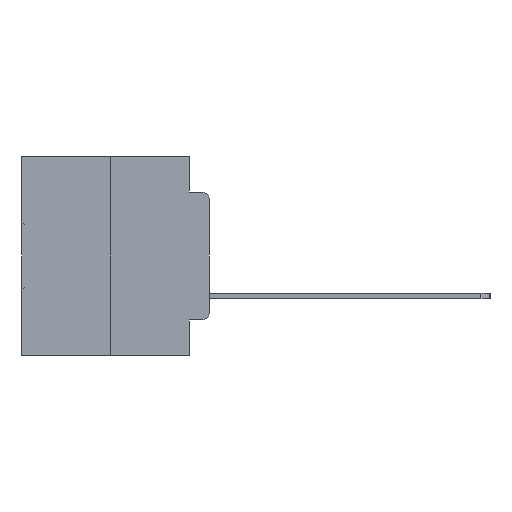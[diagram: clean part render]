
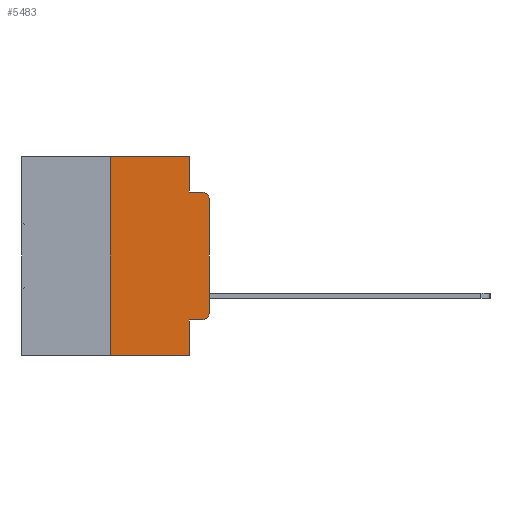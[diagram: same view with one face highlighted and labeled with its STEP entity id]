
A CAD part, left-side view. The second image highlights one B-rep face of the part: STEP entity #5483.
In plain terms, the highlighted planar face has unit normal (-1, 0, 0).
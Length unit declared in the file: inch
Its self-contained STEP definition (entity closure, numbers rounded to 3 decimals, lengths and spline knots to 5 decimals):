
#379 = DIRECTION ( 'NONE',  ( 0., 0., 1. ) ) ;
#592 = ORIENTED_EDGE ( 'NONE', *, *, #28308, .F. ) ;
#1482 = VERTEX_POINT ( 'NONE', #16239 ) ;
#1504 = VECTOR ( 'NONE', #26684, 39.37008 ) ;
#1857 = CARTESIAN_POINT ( 'NONE',  ( 0., 0.25, 0. ) ) ;
#3436 = VECTOR ( 'NONE', #13293, 39.37008 ) ;
#3845 = VECTOR ( 'NONE', #379, 39.37008 ) ;
#4010 = CARTESIAN_POINT ( 'NONE',  ( 0., 0.051, -0.4115 ) ) ;
#4102 = ORIENTED_EDGE ( 'NONE', *, *, #18301, .T. ) ;
#4181 = CARTESIAN_POINT ( 'NONE',  ( 0., 0.473, -0.5 ) ) ;
#4289 = AXIS2_PLACEMENT_3D ( 'NONE', #13052, #29774, #15468 ) ;
#4316 = VERTEX_POINT ( 'NONE', #24031 ) ;
#4359 = EDGE_CURVE ( 'NONE', #24168, #29425, #23856, .T. ) ;
#4875 = PLANE ( 'NONE',  #23037 ) ;
#5258 = VECTOR ( 'NONE', #10663, 39.37008 ) ;
#5371 = LINE ( 'NONE', #11793, #17595 ) ;
#5483 = ADVANCED_FACE ( 'NONE', ( #25859 ), #4875, .F. ) ;
#6057 = EDGE_CURVE ( 'NONE', #1482, #29607, #23603, .T. ) ;
#6245 = EDGE_CURVE ( 'NONE', #4316, #14714, #10385, .T. ) ;
#7297 = CARTESIAN_POINT ( 'NONE',  ( 0., 0.051, -0.5 ) ) ;
#7557 = ORIENTED_EDGE ( 'NONE', *, *, #7848, .T. ) ;
#7736 = CARTESIAN_POINT ( 'NONE',  ( 0., 0.25, 0. ) ) ;
#7848 = EDGE_CURVE ( 'NONE', #23346, #29607, #15579, .T. ) ;
#9597 = CARTESIAN_POINT ( 'NONE',  ( 0., 0.051, -0.0885 ) ) ;
#9608 = CARTESIAN_POINT ( 'NONE',  ( 0., 0.02, -0.1085 ) ) ;
#9739 = EDGE_LOOP ( 'NONE', ( #4102, #7557, #12170, #11010, #592, #30859, #26072, #15923, #17452, #18971 ) ) ;
#9835 = DIRECTION ( 'NONE',  ( 1., 0., 0. ) ) ;
#10385 = LINE ( 'NONE', #7736, #3845 ) ;
#10663 = DIRECTION ( 'NONE',  ( 0., -1., 0. ) ) ;
#10708 = CARTESIAN_POINT ( 'NONE',  ( 0., 0., -0.1085 ) ) ;
#10849 = CARTESIAN_POINT ( 'NONE',  ( 0., 0., 0. ) ) ;
#11010 = ORIENTED_EDGE ( 'NONE', *, *, #14440, .F. ) ;
#11793 = CARTESIAN_POINT ( 'NONE',  ( 0., 0.473, 0. ) ) ;
#11798 = AXIS2_PLACEMENT_3D ( 'NONE', #9608, #26420, #12046 ) ;
#12046 = DIRECTION ( 'NONE',  ( 0., 0., -1. ) ) ;
#12170 = ORIENTED_EDGE ( 'NONE', *, *, #6057, .F. ) ;
#12896 = EDGE_CURVE ( 'NONE', #4316, #21151, #26655, .T. ) ;
#13052 = CARTESIAN_POINT ( 'NONE',  ( 0., 0.02, -0.3915 ) ) ;
#13169 = VERTEX_POINT ( 'NONE', #29481 ) ;
#13293 = DIRECTION ( 'NONE',  ( 0., 0., 1. ) ) ;
#13726 = CARTESIAN_POINT ( 'NONE',  ( 0., 0.02, -0.4115 ) ) ;
#14221 = DIRECTION ( 'NONE',  ( 0., -1., 0. ) ) ;
#14440 = EDGE_CURVE ( 'NONE', #13169, #1482, #29871, .T. ) ;
#14623 = CARTESIAN_POINT ( 'NONE',  ( 0., 0.051, 0. ) ) ;
#14714 = VERTEX_POINT ( 'NONE', #1857 ) ;
#15455 = DIRECTION ( 'NONE',  ( 0., 0., -1. ) ) ;
#15468 = DIRECTION ( 'NONE',  ( 0., 0., -1. ) ) ;
#15579 = CIRCLE ( 'NONE', #11798, 0.02 ) ;
#15923 = ORIENTED_EDGE ( 'NONE', *, *, #28418, .F. ) ;
#16239 = CARTESIAN_POINT ( 'NONE',  ( 0., 0.051, -0.0885 ) ) ;
#17452 = ORIENTED_EDGE ( 'NONE', *, *, #4359, .T. ) ;
#17595 = VECTOR ( 'NONE', #14221, 39.37008 ) ;
#18301 = EDGE_CURVE ( 'NONE', #28210, #23346, #22806, .T. ) ;
#18928 = CIRCLE ( 'NONE', #4289, 0.02 ) ;
#18971 = ORIENTED_EDGE ( 'NONE', *, *, #24869, .T. ) ;
#19233 = DIRECTION ( 'NONE',  ( 0., -1., 0. ) ) ;
#19345 = CARTESIAN_POINT ( 'NONE',  ( 0., 0.02, -0.0885 ) ) ;
#21151 = VERTEX_POINT ( 'NONE', #7297 ) ;
#21729 = LINE ( 'NONE', #14623, #1504 ) ;
#21826 = VECTOR ( 'NONE', #30698, 39.37008 ) ;
#22806 = LINE ( 'NONE', #10849, #3436 ) ;
#23037 = AXIS2_PLACEMENT_3D ( 'NONE', #28943, #9835, #26649 ) ;
#23346 = VERTEX_POINT ( 'NONE', #10708 ) ;
#23591 = VECTOR ( 'NONE', #15455, 39.37008 ) ;
#23603 = LINE ( 'NONE', #9597, #29173 ) ;
#23856 = LINE ( 'NONE', #28181, #5258 ) ;
#24031 = CARTESIAN_POINT ( 'NONE',  ( 0., 0.25, -0.5 ) ) ;
#24168 = VERTEX_POINT ( 'NONE', #4010 ) ;
#24869 = EDGE_CURVE ( 'NONE', #29425, #28210, #18928, .T. ) ;
#25859 = FACE_OUTER_BOUND ( 'NONE', #9739, .T. ) ;
#26072 = ORIENTED_EDGE ( 'NONE', *, *, #12896, .T. ) ;
#26420 = DIRECTION ( 'NONE',  ( -1., 0., 0. ) ) ;
#26649 = DIRECTION ( 'NONE',  ( 0., 0., -1. ) ) ;
#26655 = LINE ( 'NONE', #4181, #21826 ) ;
#26684 = DIRECTION ( 'NONE',  ( 0., 0., -1. ) ) ;
#28181 = CARTESIAN_POINT ( 'NONE',  ( 0., 0.051, -0.4115 ) ) ;
#28210 = VERTEX_POINT ( 'NONE', #30595 ) ;
#28308 = EDGE_CURVE ( 'NONE', #14714, #13169, #5371, .T. ) ;
#28418 = EDGE_CURVE ( 'NONE', #24168, #21151, #21729, .T. ) ;
#28943 = CARTESIAN_POINT ( 'NONE',  ( 0., 0.473, 0. ) ) ;
#29173 = VECTOR ( 'NONE', #19233, 39.37008 ) ;
#29425 = VERTEX_POINT ( 'NONE', #13726 ) ;
#29481 = CARTESIAN_POINT ( 'NONE',  ( 0., 0.051, 0. ) ) ;
#29607 = VERTEX_POINT ( 'NONE', #19345 ) ;
#29767 = CARTESIAN_POINT ( 'NONE',  ( 0., 0.051, 0. ) ) ;
#29774 = DIRECTION ( 'NONE',  ( -1., 0., 0. ) ) ;
#29871 = LINE ( 'NONE', #29767, #23591 ) ;
#30595 = CARTESIAN_POINT ( 'NONE',  ( 0., 0., -0.3915 ) ) ;
#30698 = DIRECTION ( 'NONE',  ( 0., -1., 0. ) ) ;
#30859 = ORIENTED_EDGE ( 'NONE', *, *, #6245, .F. ) ;
